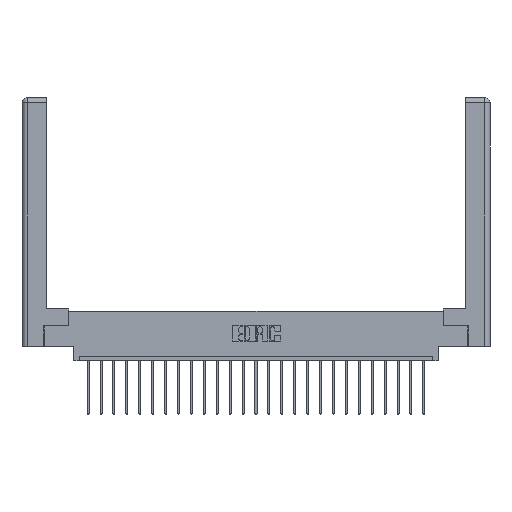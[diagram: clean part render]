
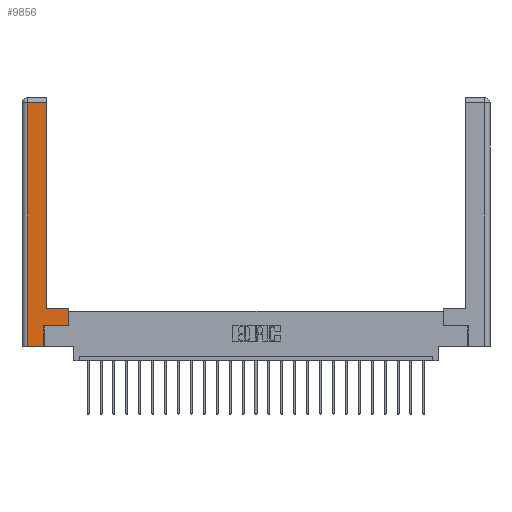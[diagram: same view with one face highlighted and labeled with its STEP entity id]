
A CAD part, top view. The second image highlights one B-rep face of the part: STEP entity #9856.
In plain terms, the highlighted planar face has unit normal (0, 0, 1).
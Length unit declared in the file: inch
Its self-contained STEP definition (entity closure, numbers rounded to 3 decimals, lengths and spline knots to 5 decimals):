
#98 = VERTEX_POINT ( 'NONE', #5490 ) ;
#810 = CARTESIAN_POINT ( 'NONE',  ( 0.265, 0., 0. ) ) ;
#887 = DIRECTION ( 'NONE',  ( 1., 0., 0. ) ) ;
#1618 = ORIENTED_EDGE ( 'NONE', *, *, #24487, .T. ) ;
#2759 = VERTEX_POINT ( 'NONE', #10237 ) ;
#2764 = EDGE_CURVE ( 'NONE', #2759, #98, #15955, .T. ) ;
#3043 = ORIENTED_EDGE ( 'NONE', *, *, #3385, .T. ) ;
#3284 = LINE ( 'NONE', #810, #13161 ) ;
#3385 = EDGE_CURVE ( 'NONE', #9385, #22722, #5431, .T. ) ;
#3611 = VECTOR ( 'NONE', #23476, 39.37008 ) ;
#4119 = EDGE_CURVE ( 'NONE', #14417, #9385, #23108, .T. ) ;
#4594 = DIRECTION ( 'NONE',  ( -1., 0., 0. ) ) ;
#5431 = LINE ( 'NONE', #16337, #17116 ) ;
#5490 = CARTESIAN_POINT ( 'NONE',  ( 0.265, 0.245, 0. ) ) ;
#5546 = CARTESIAN_POINT ( 'NONE',  ( 0.565, 0.245, 0. ) ) ;
#5672 = PLANE ( 'NONE',  #6662 ) ;
#6321 = DIRECTION ( 'NONE',  ( 0., -1., 0. ) ) ;
#6332 = EDGE_LOOP ( 'NONE', ( #23589, #1618, #23103, #13659, #7392, #12631, #24668, #3043 ) ) ;
#6501 = VERTEX_POINT ( 'NONE', #12699 ) ;
#6662 = AXIS2_PLACEMENT_3D ( 'NONE', #11226, #9316, #13334 ) ;
#6779 = VECTOR ( 'NONE', #4594, 39.37008 ) ;
#6966 = LINE ( 'NONE', #15958, #12916 ) ;
#7358 = LINE ( 'NONE', #11602, #6779 ) ;
#7392 = ORIENTED_EDGE ( 'NONE', *, *, #2764, .T. ) ;
#8587 = EDGE_CURVE ( 'NONE', #6501, #10375, #6966, .T. ) ;
#9233 = EDGE_CURVE ( 'NONE', #98, #14417, #21023, .T. ) ;
#9316 = DIRECTION ( 'NONE',  ( 0., 0., -1. ) ) ;
#9385 = VERTEX_POINT ( 'NONE', #17532 ) ;
#9856 = ADVANCED_FACE ( 'NONE', ( #17634 ), #5672, .F. ) ;
#10237 = CARTESIAN_POINT ( 'NONE',  ( 0.265, 0., 0. ) ) ;
#10375 = VERTEX_POINT ( 'NONE', #14929 ) ;
#11054 = CARTESIAN_POINT ( 'NONE',  ( 0.295, 2.94, 0. ) ) ;
#11226 = CARTESIAN_POINT ( 'NONE',  ( 0., 0., 0. ) ) ;
#11288 = VERTEX_POINT ( 'NONE', #11054 ) ;
#11602 = CARTESIAN_POINT ( 'NONE',  ( 0.0615, 2.94, 0. ) ) ;
#12218 = LINE ( 'NONE', #16828, #16767 ) ;
#12494 = DIRECTION ( 'NONE',  ( -1., 0., 0. ) ) ;
#12631 = ORIENTED_EDGE ( 'NONE', *, *, #9233, .T. ) ;
#12699 = CARTESIAN_POINT ( 'NONE',  ( 0.0615, 2.94, 0. ) ) ;
#12838 = VECTOR ( 'NONE', #23202, 39.37008 ) ;
#12916 = VECTOR ( 'NONE', #6321, 39.37008 ) ;
#13161 = VECTOR ( 'NONE', #887, 39.37008 ) ;
#13197 = CARTESIAN_POINT ( 'NONE',  ( 0.565, 0.245, 0. ) ) ;
#13334 = DIRECTION ( 'NONE',  ( -1., 0., 0. ) ) ;
#13659 = ORIENTED_EDGE ( 'NONE', *, *, #22546, .T. ) ;
#14245 = CARTESIAN_POINT ( 'NONE',  ( 0.295, 0.45, 0. ) ) ;
#14417 = VERTEX_POINT ( 'NONE', #13197 ) ;
#14929 = CARTESIAN_POINT ( 'NONE',  ( 0.0615, 0., 0. ) ) ;
#15831 = CARTESIAN_POINT ( 'NONE',  ( 0.565, 0.45, 0. ) ) ;
#15955 = LINE ( 'NONE', #21422, #21333 ) ;
#15958 = CARTESIAN_POINT ( 'NONE',  ( 0.0615, 0., 0. ) ) ;
#16337 = CARTESIAN_POINT ( 'NONE',  ( 0.295, 0.45, 0. ) ) ;
#16767 = VECTOR ( 'NONE', #20683, 39.37008 ) ;
#16828 = CARTESIAN_POINT ( 'NONE',  ( 0.295, 3., 0. ) ) ;
#17116 = VECTOR ( 'NONE', #12494, 39.37008 ) ;
#17532 = CARTESIAN_POINT ( 'NONE',  ( 0.565, 0.45, 0. ) ) ;
#17634 = FACE_OUTER_BOUND ( 'NONE', #6332, .T. ) ;
#19915 = DIRECTION ( 'NONE',  ( 0., 1., 0. ) ) ;
#20683 = DIRECTION ( 'NONE',  ( 0., 1., 0. ) ) ;
#21023 = LINE ( 'NONE', #5546, #3611 ) ;
#21333 = VECTOR ( 'NONE', #19915, 39.37008 ) ;
#21422 = CARTESIAN_POINT ( 'NONE',  ( 0.265, 0.245, 0. ) ) ;
#22546 = EDGE_CURVE ( 'NONE', #10375, #2759, #3284, .T. ) ;
#22722 = VERTEX_POINT ( 'NONE', #14245 ) ;
#23103 = ORIENTED_EDGE ( 'NONE', *, *, #8587, .T. ) ;
#23108 = LINE ( 'NONE', #15831, #12838 ) ;
#23202 = DIRECTION ( 'NONE',  ( 0., 1., 0. ) ) ;
#23303 = EDGE_CURVE ( 'NONE', #22722, #11288, #12218, .T. ) ;
#23476 = DIRECTION ( 'NONE',  ( 1., 0., 0. ) ) ;
#23589 = ORIENTED_EDGE ( 'NONE', *, *, #23303, .T. ) ;
#24487 = EDGE_CURVE ( 'NONE', #11288, #6501, #7358, .T. ) ;
#24668 = ORIENTED_EDGE ( 'NONE', *, *, #4119, .T. ) ;
